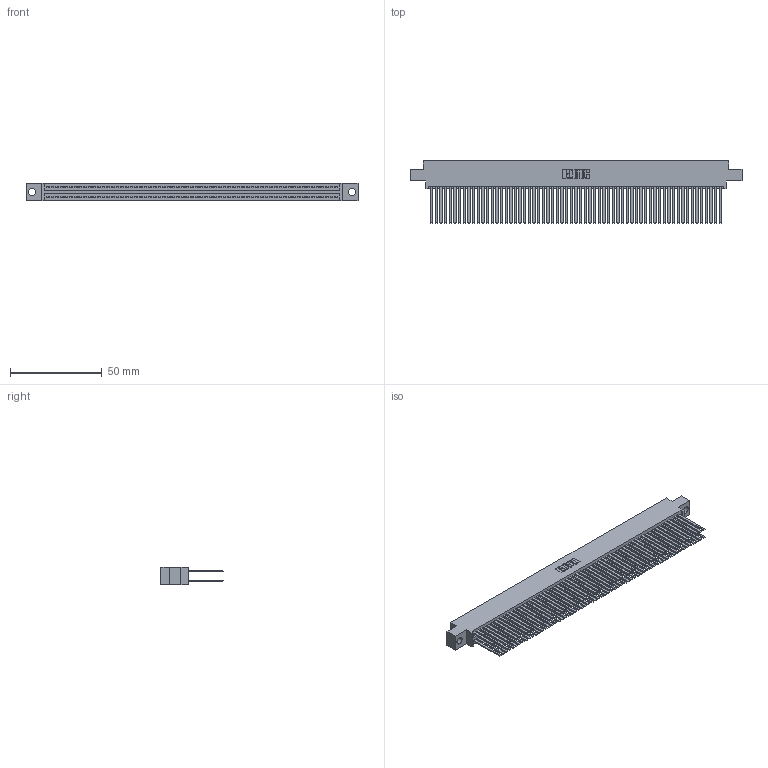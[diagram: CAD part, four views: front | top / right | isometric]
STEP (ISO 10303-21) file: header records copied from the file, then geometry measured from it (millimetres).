
FILE_DESCRIPTION (( 'STEP AP203' ), '1' );
FILE_NAME ('395-126-544-804.STEP', '2021-06-17T23:00:56', ( '' ), ( '' ), 'SwSTEP 2.0', 'SolidWorks 2020', '' );
FILE_SCHEMA (( 'CONFIG_CONTROL_DESIGN' ));
Length unit declared in the file: inch
Products named in the file (3): 345 Part_0.170 Offset - 0.156 Dia-TI; 395-126-544-804; 345-292-001_345-293-144
Assembly tree (127 placements, depth 2):
  395-126-544-804
    345 Part_0.170 Offset - 0.156 Dia-TI
    345-292-001_345-293-144  x126
Bounding box: 181.23 x 33.96 x 9.4 mm (x, y, z)
Volume: 19346.7 mm3; surface area: 34176.2 mm2
Topology: 127 solids, 127 shells, 5688 faces, 16895 edges, 11094 vertices
Faces by surface type: plane 3752, cylinder 1936
Entity records: 46971 total; most frequent: CARTESIAN_POINT 7858, ORIENTED_EDGE 7790, DIRECTION 6899, EDGE_CURVE 3895, VECTOR 3515, LINE 3515, VERTEX_POINT 2594, AXIS2_PLACEMENT_3D 1692
